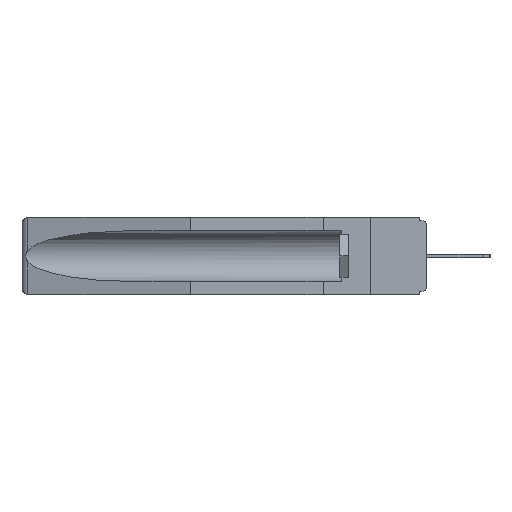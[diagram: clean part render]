
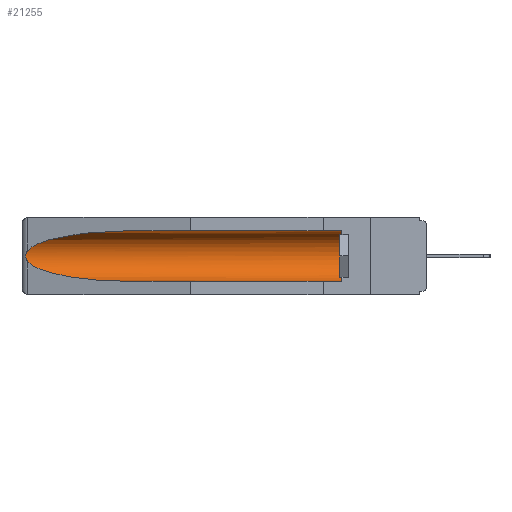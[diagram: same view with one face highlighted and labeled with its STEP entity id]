
A CAD part, left-side view. The second image highlights one B-rep face of the part: STEP entity #21255.
In plain terms, the highlighted cylindrical face has radius 2.857 mm (diameter 5.715 mm), a partial arc.
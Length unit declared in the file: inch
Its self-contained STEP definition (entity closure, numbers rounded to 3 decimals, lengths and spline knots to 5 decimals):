
#665 = EDGE_CURVE ( 'NONE', #24169, #16018, #14450, .T. ) ;
#1702 = CARTESIAN_POINT ( 'NONE',  ( 0.26537, 1.52718, -0.19328 ) ) ;
#1870 = CYLINDRICAL_SURFACE ( 'NONE', #13251, 0.1125 ) ;
#2478 = VERTEX_POINT ( 'NONE', #1702 ) ;
#2520 = ORIENTED_EDGE ( 'NONE', *, *, #19673, .T. ) ;
#2853 = EDGE_LOOP ( 'NONE', ( #2520, #4443, #17168, #9375, #7698, #6412 ) ) ;
#2963 = CARTESIAN_POINT ( 'NONE',  ( 0.155, -0.30754, -0.059 ) ) ;
#3103 = CARTESIAN_POINT ( 'NONE',  ( 0.26537, 1.52718, -0.19328 ) ) ;
#3157 = DIRECTION ( 'NONE',  ( 0., 1., 0. ) ) ;
#4229 = VECTOR ( 'NONE', #12466, 39.37008 ) ;
#4443 = ORIENTED_EDGE ( 'NONE', *, *, #7170, .T. ) ;
#4861 = FACE_OUTER_BOUND ( 'NONE', #2853, .T. ) ;
#5035 = CARTESIAN_POINT ( 'NONE',  ( 0.155, -0.30754, -0.284 ) ) ;
#5740 = CARTESIAN_POINT ( 'NONE',  ( 0.155, 1.07973, -0.059 ) ) ;
#5936 = CARTESIAN_POINT ( 'NONE',  ( 0.155, 1.07973, -0.059 ) ) ;
#6065 = CARTESIAN_POINT ( 'NONE',  ( 0.2673, 1.5327, -0.16383 ) ) ;
#6412 = ORIENTED_EDGE ( 'NONE', *, *, #665, .T. ) ;
#6652 = VECTOR ( 'NONE', #3157, 39.37008 ) ;
#7170 = EDGE_CURVE ( 'NONE', #22324, #2478, #10159, .T. ) ;
#7391 = AXIS2_PLACEMENT_3D ( 'NONE', #23082, #11539, #9679 ) ;
#7698 = ORIENTED_EDGE ( 'NONE', *, *, #17000, .T. ) ;
#8826 = DIRECTION ( 'NONE',  ( 0., 1., 0. ) ) ;
#9066 = EDGE_CURVE ( 'NONE', #2478, #10528, #18353, .T. ) ;
#9213 = CARTESIAN_POINT ( 'NONE',  ( 0.155, 1.07973, -0.284 ) ) ;
#9375 = ORIENTED_EDGE ( 'NONE', *, *, #17803, .F. ) ;
#9679 = DIRECTION ( 'NONE',  ( 0., 0., 1. ) ) ;
#9708 =( BOUNDED_CURVE ( )  B_SPLINE_CURVE ( 3, ( #5740, #11542, #13480, #15424 ),
 .UNSPECIFIED., .F., .F. ) 
 B_SPLINE_CURVE_WITH_KNOTS ( ( 4, 4 ),
 ( 4.71239, 6.08839 ),
 .UNSPECIFIED. ) 
 CURVE ( )  GEOMETRIC_REPRESENTATION_ITEM ( )  RATIONAL_B_SPLINE_CURVE ( ( 1., 0.848, 0.848, 1. ) ) 
 REPRESENTATION_ITEM ( '' )  );
#9775 = CARTESIAN_POINT ( 'NONE',  ( 0.26537, 1.52718, -0.14972 ) ) ;
#10014 = CARTESIAN_POINT ( 'NONE',  ( 0.2675, 1.53308, -0.17534 ) ) ;
#10159 = B_SPLINE_CURVE_WITH_KNOTS ( 'NONE', 3,
 ( #9775, #17863, #17625, #6065, #15761, #10014, #12024, #18521, #10675, #3103 ),
 .UNSPECIFIED., .F., .F.,
 ( 4, 2, 2, 2, 4 ),
 ( 0., 0.00029, 0.00058, 0.00087, 0.00117 ),
 .UNSPECIFIED. ) ;
#10335 = CARTESIAN_POINT ( 'NONE',  ( 0.26537, 1.52718, -0.14972 ) ) ;
#10528 = VERTEX_POINT ( 'NONE', #10915 ) ;
#10675 = CARTESIAN_POINT ( 'NONE',  ( 0.26597, 1.5296, -0.19026 ) ) ;
#10915 = CARTESIAN_POINT ( 'NONE',  ( 0.155, 1.07973, -0.284 ) ) ;
#11069 = CARTESIAN_POINT ( 'NONE',  ( 0.25451, 1.48313, -0.24835 ) ) ;
#11539 = DIRECTION ( 'NONE',  ( 0., -1., 0. ) ) ;
#11542 = CARTESIAN_POINT ( 'NONE',  ( 0.21114, 1.30732, -0.059 ) ) ;
#12024 = CARTESIAN_POINT ( 'NONE',  ( 0.2673, 1.53269, -0.17917 ) ) ;
#12466 = DIRECTION ( 'NONE',  ( 0., 1., 0. ) ) ;
#12794 = CARTESIAN_POINT ( 'NONE',  ( 0.155, -0.30754, -0.1715 ) ) ;
#13251 = AXIS2_PLACEMENT_3D ( 'NONE', #12794, #8826, #20225 ) ;
#13480 = CARTESIAN_POINT ( 'NONE',  ( 0.25451, 1.48313, -0.09465 ) ) ;
#13813 = VERTEX_POINT ( 'NONE', #20645 ) ;
#14208 = CARTESIAN_POINT ( 'NONE',  ( 0.155, 0.126, -0.059 ) ) ;
#14450 = LINE ( 'NONE', #2963, #4229 ) ;
#15424 = CARTESIAN_POINT ( 'NONE',  ( 0.26537, 1.52718, -0.14972 ) ) ;
#15761 = CARTESIAN_POINT ( 'NONE',  ( 0.2675, 1.53308, -0.16763 ) ) ;
#16018 = VERTEX_POINT ( 'NONE', #5936 ) ;
#17000 = EDGE_CURVE ( 'NONE', #13813, #24169, #24471, .T. ) ;
#17168 = ORIENTED_EDGE ( 'NONE', *, *, #9066, .T. ) ;
#17625 = CARTESIAN_POINT ( 'NONE',  ( 0.26654, 1.53092, -0.15636 ) ) ;
#17803 = EDGE_CURVE ( 'NONE', #13813, #10528, #24125, .T. ) ;
#17863 = CARTESIAN_POINT ( 'NONE',  ( 0.26597, 1.52961, -0.15275 ) ) ;
#18353 =( BOUNDED_CURVE ( )  B_SPLINE_CURVE ( 3, ( #21019, #11069, #20780, #9213 ),
 .UNSPECIFIED., .F., .F. ) 
 B_SPLINE_CURVE_WITH_KNOTS ( ( 4, 4 ),
 ( 0.1948, 1.5708 ),
 .UNSPECIFIED. ) 
 CURVE ( )  GEOMETRIC_REPRESENTATION_ITEM ( )  RATIONAL_B_SPLINE_CURVE ( ( 1., 0.848, 0.848, 1. ) ) 
 REPRESENTATION_ITEM ( '' )  );
#18521 = CARTESIAN_POINT ( 'NONE',  ( 0.26655, 1.53094, -0.18657 ) ) ;
#19673 = EDGE_CURVE ( 'NONE', #16018, #22324, #9708, .T. ) ;
#20225 = DIRECTION ( 'NONE',  ( 0., 0., 1. ) ) ;
#20645 = CARTESIAN_POINT ( 'NONE',  ( 0.155, 0.126, -0.284 ) ) ;
#20780 = CARTESIAN_POINT ( 'NONE',  ( 0.21114, 1.30732, -0.284 ) ) ;
#21019 = CARTESIAN_POINT ( 'NONE',  ( 0.26537, 1.52718, -0.19328 ) ) ;
#21255 = ADVANCED_FACE ( 'NONE', ( #4861 ), #1870, .F. ) ;
#22324 = VERTEX_POINT ( 'NONE', #10335 ) ;
#23082 = CARTESIAN_POINT ( 'NONE',  ( 0.155, 0.126, -0.1715 ) ) ;
#24125 = LINE ( 'NONE', #5035, #6652 ) ;
#24169 = VERTEX_POINT ( 'NONE', #14208 ) ;
#24471 = CIRCLE ( 'NONE', #7391, 0.1125 ) ;
